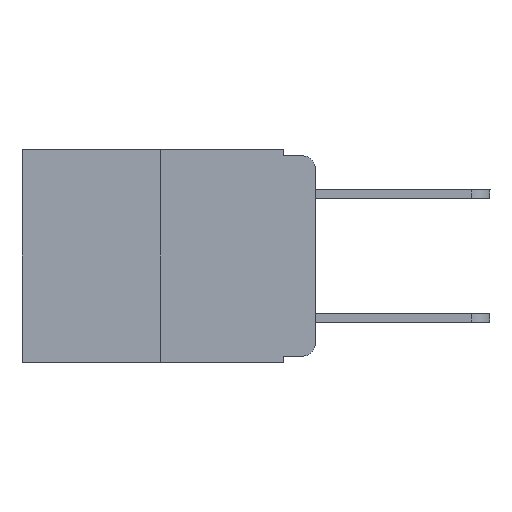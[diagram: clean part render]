
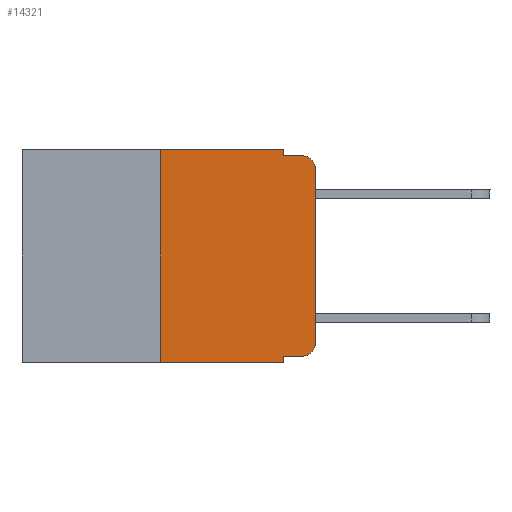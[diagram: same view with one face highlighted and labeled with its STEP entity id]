
A CAD part, left-side view. The second image highlights one B-rep face of the part: STEP entity #14321.
In plain terms, the highlighted planar face has unit normal (-1, 0, 0).
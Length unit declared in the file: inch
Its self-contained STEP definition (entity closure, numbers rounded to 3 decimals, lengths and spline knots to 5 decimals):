
#25 = CARTESIAN_POINT ( 'NONE',  ( 0., 0.051, 0. ) ) ;
#692 = CARTESIAN_POINT ( 'NONE',  ( 0., 0., 0. ) ) ;
#883 = VERTEX_POINT ( 'NONE', #1181 ) ;
#931 = CARTESIAN_POINT ( 'NONE',  ( 0., 0.25, -0.343 ) ) ;
#1181 = CARTESIAN_POINT ( 'NONE',  ( 0., 0.051, -0.343 ) ) ;
#1282 = DIRECTION ( 'NONE',  ( 0., 0., -1. ) ) ;
#2240 = VECTOR ( 'NONE', #3760, 39.37008 ) ;
#2411 = ORIENTED_EDGE ( 'NONE', *, *, #19775, .F. ) ;
#2501 = EDGE_CURVE ( 'NONE', #4780, #883, #15791, .T. ) ;
#2704 = AXIS2_PLACEMENT_3D ( 'NONE', #19994, #2908, #13935 ) ;
#2908 = DIRECTION ( 'NONE',  ( 1., 0., 0. ) ) ;
#2924 = VERTEX_POINT ( 'NONE', #3002 ) ;
#3002 = CARTESIAN_POINT ( 'NONE',  ( 0., 0., -0.313 ) ) ;
#3067 = VERTEX_POINT ( 'NONE', #16305 ) ;
#3125 = DIRECTION ( 'NONE',  ( 0., -1., 0. ) ) ;
#3364 = AXIS2_PLACEMENT_3D ( 'NONE', #18516, #12205, #20069 ) ;
#3528 = LINE ( 'NONE', #6980, #3683 ) ;
#3683 = VECTOR ( 'NONE', #13139, 39.37008 ) ;
#3760 = DIRECTION ( 'NONE',  ( 0., -1., 0. ) ) ;
#3970 = CIRCLE ( 'NONE', #3364, 0.02 ) ;
#4439 = PLANE ( 'NONE',  #2704 ) ;
#4475 = VECTOR ( 'NONE', #3125, 39.37008 ) ;
#4780 = VERTEX_POINT ( 'NONE', #931 ) ;
#5212 = LINE ( 'NONE', #692, #16641 ) ;
#6073 = CARTESIAN_POINT ( 'NONE',  ( 0., 0., -0.03 ) ) ;
#6272 = AXIS2_PLACEMENT_3D ( 'NONE', #19445, #15779, #18744 ) ;
#6293 = CARTESIAN_POINT ( 'NONE',  ( 0., 0.051, 0. ) ) ;
#6304 = ORIENTED_EDGE ( 'NONE', *, *, #16559, .F. ) ;
#6409 = VECTOR ( 'NONE', #10754, 39.37008 ) ;
#6702 = DIRECTION ( 'NONE',  ( 0., -1., 0. ) ) ;
#6896 = DIRECTION ( 'NONE',  ( 0., 0., 1. ) ) ;
#6980 = CARTESIAN_POINT ( 'NONE',  ( 0., 0.051, -0.333 ) ) ;
#7490 = EDGE_CURVE ( 'NONE', #4780, #9775, #12847, .T. ) ;
#7990 = LINE ( 'NONE', #6293, #6409 ) ;
#8028 = ORIENTED_EDGE ( 'NONE', *, *, #14145, .T. ) ;
#8309 = LINE ( 'NONE', #18787, #2240 ) ;
#8865 = CARTESIAN_POINT ( 'NONE',  ( 0., 0.25, 0. ) ) ;
#9008 = ORIENTED_EDGE ( 'NONE', *, *, #12572, .F. ) ;
#9177 = CIRCLE ( 'NONE', #6272, 0.02 ) ;
#9775 = VERTEX_POINT ( 'NONE', #8865 ) ;
#9870 = DIRECTION ( 'NONE',  ( 0., 0., 1. ) ) ;
#10510 = EDGE_CURVE ( 'NONE', #9775, #17802, #8309, .T. ) ;
#10754 = DIRECTION ( 'NONE',  ( 0., 0., -1. ) ) ;
#10934 = LINE ( 'NONE', #25, #17535 ) ;
#11197 = CARTESIAN_POINT ( 'NONE',  ( 0., 0.02, -0.01 ) ) ;
#12205 = DIRECTION ( 'NONE',  ( -1., 0., 0. ) ) ;
#12375 = CARTESIAN_POINT ( 'NONE',  ( 0., 0.051, 0. ) ) ;
#12404 = VECTOR ( 'NONE', #6896, 39.37008 ) ;
#12572 = EDGE_CURVE ( 'NONE', #17802, #20107, #10934, .T. ) ;
#12847 = LINE ( 'NONE', #19080, #12404 ) ;
#13029 = VERTEX_POINT ( 'NONE', #6073 ) ;
#13139 = DIRECTION ( 'NONE',  ( 0., -1., 0. ) ) ;
#13257 = ORIENTED_EDGE ( 'NONE', *, *, #16205, .T. ) ;
#13311 = ORIENTED_EDGE ( 'NONE', *, *, #14840, .T. ) ;
#13650 = FACE_OUTER_BOUND ( 'NONE', #17515, .T. ) ;
#13797 = CARTESIAN_POINT ( 'NONE',  ( 0., 0.051, -0.01 ) ) ;
#13935 = DIRECTION ( 'NONE',  ( 0., 0., -1. ) ) ;
#14145 = EDGE_CURVE ( 'NONE', #3067, #19945, #3528, .T. ) ;
#14321 = ADVANCED_FACE ( 'NONE', ( #13650 ), #4439, .F. ) ;
#14769 = CARTESIAN_POINT ( 'NONE',  ( 0., 0.051, -0.01 ) ) ;
#14840 = EDGE_CURVE ( 'NONE', #13029, #17285, #3970, .T. ) ;
#15131 = ORIENTED_EDGE ( 'NONE', *, *, #7490, .F. ) ;
#15592 = EDGE_CURVE ( 'NONE', #19945, #2924, #9177, .T. ) ;
#15719 = LINE ( 'NONE', #13797, #18290 ) ;
#15779 = DIRECTION ( 'NONE',  ( -1., 0., 0. ) ) ;
#15791 = LINE ( 'NONE', #17033, #4475 ) ;
#16199 = CARTESIAN_POINT ( 'NONE',  ( 0., 0.02, -0.333 ) ) ;
#16205 = EDGE_CURVE ( 'NONE', #2924, #13029, #5212, .T. ) ;
#16305 = CARTESIAN_POINT ( 'NONE',  ( 0., 0.051, -0.333 ) ) ;
#16546 = ORIENTED_EDGE ( 'NONE', *, *, #2501, .T. ) ;
#16559 = EDGE_CURVE ( 'NONE', #20107, #17285, #15719, .T. ) ;
#16641 = VECTOR ( 'NONE', #9870, 39.37008 ) ;
#17033 = CARTESIAN_POINT ( 'NONE',  ( 0., 0.473, -0.343 ) ) ;
#17285 = VERTEX_POINT ( 'NONE', #11197 ) ;
#17515 = EDGE_LOOP ( 'NONE', ( #13257, #13311, #6304, #9008, #17617, #15131, #16546, #2411, #8028, #18279 ) ) ;
#17535 = VECTOR ( 'NONE', #1282, 39.37008 ) ;
#17617 = ORIENTED_EDGE ( 'NONE', *, *, #10510, .F. ) ;
#17802 = VERTEX_POINT ( 'NONE', #12375 ) ;
#18279 = ORIENTED_EDGE ( 'NONE', *, *, #15592, .T. ) ;
#18290 = VECTOR ( 'NONE', #6702, 39.37008 ) ;
#18516 = CARTESIAN_POINT ( 'NONE',  ( 0., 0.02, -0.03 ) ) ;
#18744 = DIRECTION ( 'NONE',  ( 0., 0., -1. ) ) ;
#18787 = CARTESIAN_POINT ( 'NONE',  ( 0., 0.473, 0. ) ) ;
#19080 = CARTESIAN_POINT ( 'NONE',  ( 0., 0.25, 0. ) ) ;
#19445 = CARTESIAN_POINT ( 'NONE',  ( 0., 0.02, -0.313 ) ) ;
#19775 = EDGE_CURVE ( 'NONE', #3067, #883, #7990, .T. ) ;
#19945 = VERTEX_POINT ( 'NONE', #16199 ) ;
#19994 = CARTESIAN_POINT ( 'NONE',  ( 0., 0.473, 0. ) ) ;
#20069 = DIRECTION ( 'NONE',  ( 0., 0., -1. ) ) ;
#20107 = VERTEX_POINT ( 'NONE', #14769 ) ;
